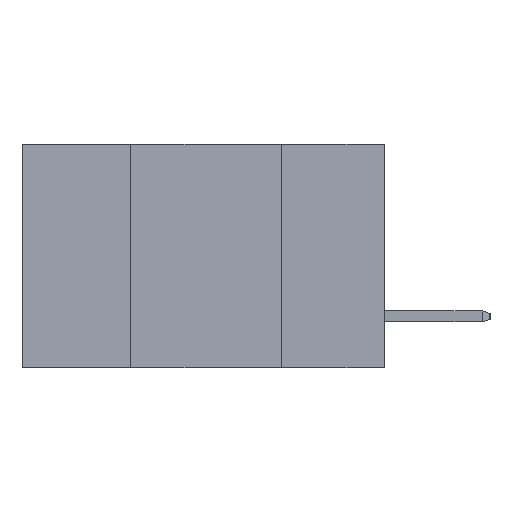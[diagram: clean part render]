
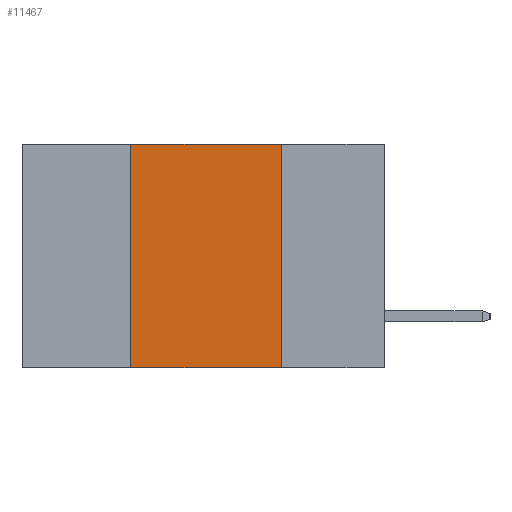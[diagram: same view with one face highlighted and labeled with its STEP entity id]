
A CAD part, left-side view. The second image highlights one B-rep face of the part: STEP entity #11467.
In plain terms, the highlighted planar face has unit normal (-1, 0, 0).
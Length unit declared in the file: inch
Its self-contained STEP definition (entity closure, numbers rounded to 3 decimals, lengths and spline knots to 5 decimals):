
#653 = LINE ( 'NONE', #22171, #30602 ) ;
#1014 = VERTEX_POINT ( 'NONE', #28862 ) ;
#1104 = FACE_OUTER_BOUND ( 'NONE', #20677, .T. ) ;
#2026 = VERTEX_POINT ( 'NONE', #7167 ) ;
#2034 = DIRECTION ( 'NONE',  ( 0., 0., -1. ) ) ;
#3591 = AXIS2_PLACEMENT_3D ( 'NONE', #9393, #20564, #2034 ) ;
#5171 = DIRECTION ( 'NONE',  ( 0., -1., 0. ) ) ;
#5986 = EDGE_CURVE ( 'NONE', #8219, #2026, #16818, .T. ) ;
#7167 = CARTESIAN_POINT ( 'NONE',  ( 0., 0.42, 0. ) ) ;
#8219 = VERTEX_POINT ( 'NONE', #28577 ) ;
#9236 = CARTESIAN_POINT ( 'NONE',  ( 0., 0.6, 0. ) ) ;
#9393 = CARTESIAN_POINT ( 'NONE',  ( 0., 0.6, 0. ) ) ;
#9541 = CARTESIAN_POINT ( 'NONE',  ( 0., 0.17, 0. ) ) ;
#9719 = PLANE ( 'NONE',  #3591 ) ;
#9784 = EDGE_CURVE ( 'NONE', #22014, #1014, #19959, .T. ) ;
#11467 = ADVANCED_FACE ( 'NONE', ( #1104 ), #9719, .F. ) ;
#15142 = VECTOR ( 'NONE', #19043, 39.37008 ) ;
#16055 = VECTOR ( 'NONE', #24577, 39.37008 ) ;
#16398 = EDGE_CURVE ( 'NONE', #8219, #1014, #653, .T. ) ;
#16818 = LINE ( 'NONE', #22838, #16055 ) ;
#18927 = CARTESIAN_POINT ( 'NONE',  ( 0., 0.17, 0. ) ) ;
#19043 = DIRECTION ( 'NONE',  ( 0., -1., 0. ) ) ;
#19542 = ORIENTED_EDGE ( 'NONE', *, *, #5986, .F. ) ;
#19959 = LINE ( 'NONE', #18927, #26345 ) ;
#20564 = DIRECTION ( 'NONE',  ( 1., 0., 0. ) ) ;
#20653 = EDGE_CURVE ( 'NONE', #2026, #22014, #27942, .T. ) ;
#20677 = EDGE_LOOP ( 'NONE', ( #21323, #23205, #19542, #26893 ) ) ;
#21323 = ORIENTED_EDGE ( 'NONE', *, *, #9784, .F. ) ;
#22014 = VERTEX_POINT ( 'NONE', #9541 ) ;
#22171 = CARTESIAN_POINT ( 'NONE',  ( 0., 0.6, -0.37 ) ) ;
#22838 = CARTESIAN_POINT ( 'NONE',  ( 0., 0.42, 0. ) ) ;
#23205 = ORIENTED_EDGE ( 'NONE', *, *, #20653, .F. ) ;
#24577 = DIRECTION ( 'NONE',  ( 0., 0., 1. ) ) ;
#26345 = VECTOR ( 'NONE', #30693, 39.37008 ) ;
#26893 = ORIENTED_EDGE ( 'NONE', *, *, #16398, .T. ) ;
#27942 = LINE ( 'NONE', #9236, #15142 ) ;
#28577 = CARTESIAN_POINT ( 'NONE',  ( 0., 0.42, -0.37 ) ) ;
#28862 = CARTESIAN_POINT ( 'NONE',  ( 0., 0.17, -0.37 ) ) ;
#30602 = VECTOR ( 'NONE', #5171, 39.37008 ) ;
#30693 = DIRECTION ( 'NONE',  ( 0., 0., -1. ) ) ;
